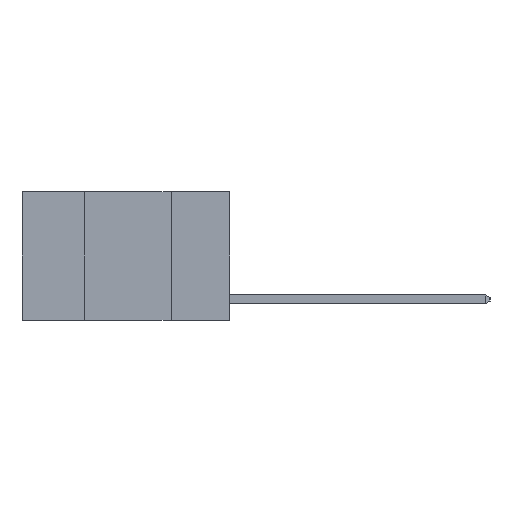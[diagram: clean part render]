
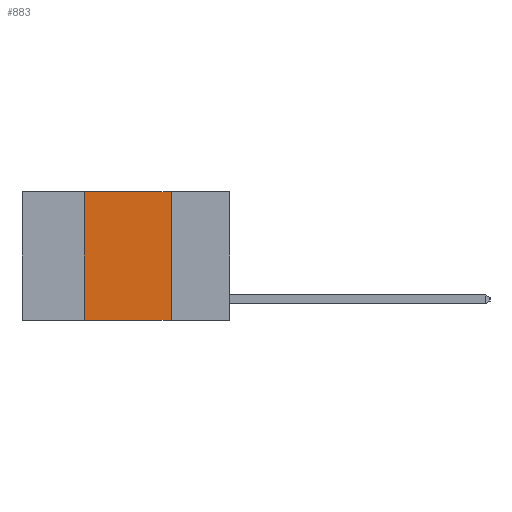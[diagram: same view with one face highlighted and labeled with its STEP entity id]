
A CAD part, left-side view. The second image highlights one B-rep face of the part: STEP entity #883.
In plain terms, the highlighted planar face has unit normal (-1, 0, 0).
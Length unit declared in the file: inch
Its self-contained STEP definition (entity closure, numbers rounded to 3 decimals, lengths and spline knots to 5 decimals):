
#25 = LINE ( 'NONE', #2860, #266 ) ;
#266 = VECTOR ( 'NONE', #7076, 39.37008 ) ;
#391 = VERTEX_POINT ( 'NONE', #4552 ) ;
#779 = CARTESIAN_POINT ( 'NONE',  ( 0., 0.17, 0. ) ) ;
#883 = ADVANCED_FACE ( 'NONE', ( #3586 ), #3807, .F. ) ;
#1099 = ORIENTED_EDGE ( 'NONE', *, *, #2950, .F. ) ;
#1114 = VERTEX_POINT ( 'NONE', #779 ) ;
#1129 = ORIENTED_EDGE ( 'NONE', *, *, #2353, .F. ) ;
#1138 = ORIENTED_EDGE ( 'NONE', *, *, #4834, .F. ) ;
#1159 = ORIENTED_EDGE ( 'NONE', *, *, #6149, .T. ) ;
#1389 = VERTEX_POINT ( 'NONE', #4564 ) ;
#2198 = AXIS2_PLACEMENT_3D ( 'NONE', #8016, #5359, #7783 ) ;
#2353 = EDGE_CURVE ( 'NONE', #5179, #1114, #6634, .T. ) ;
#2663 = VECTOR ( 'NONE', #3576, 39.37008 ) ;
#2860 = CARTESIAN_POINT ( 'NONE',  ( 0., 0.17, 0. ) ) ;
#2915 = CARTESIAN_POINT ( 'NONE',  ( 0., 0.42, 0. ) ) ;
#2950 = EDGE_CURVE ( 'NONE', #1114, #1389, #25, .T. ) ;
#3290 = CARTESIAN_POINT ( 'NONE',  ( 0., 0.42, 0. ) ) ;
#3499 = CARTESIAN_POINT ( 'NONE',  ( 0., 0.6, -0.37 ) ) ;
#3576 = DIRECTION ( 'NONE',  ( 0., 0., 1. ) ) ;
#3586 = FACE_OUTER_BOUND ( 'NONE', #4566, .T. ) ;
#3807 = PLANE ( 'NONE',  #2198 ) ;
#3913 = VECTOR ( 'NONE', #7062, 39.37008 ) ;
#4552 = CARTESIAN_POINT ( 'NONE',  ( 0., 0.42, -0.37 ) ) ;
#4564 = CARTESIAN_POINT ( 'NONE',  ( 0., 0.17, -0.37 ) ) ;
#4566 = EDGE_LOOP ( 'NONE', ( #1099, #1129, #1138, #1159 ) ) ;
#4834 = EDGE_CURVE ( 'NONE', #391, #5179, #5997, .T. ) ;
#5179 = VERTEX_POINT ( 'NONE', #3290 ) ;
#5359 = DIRECTION ( 'NONE',  ( 1., 0., 0. ) ) ;
#5884 = DIRECTION ( 'NONE',  ( 0., -1., 0. ) ) ;
#5970 = CARTESIAN_POINT ( 'NONE',  ( 0., 0.6, 0. ) ) ;
#5997 = LINE ( 'NONE', #2915, #2663 ) ;
#6149 = EDGE_CURVE ( 'NONE', #391, #1389, #7016, .T. ) ;
#6634 = LINE ( 'NONE', #5970, #7937 ) ;
#7016 = LINE ( 'NONE', #3499, #3913 ) ;
#7062 = DIRECTION ( 'NONE',  ( 0., -1., 0. ) ) ;
#7076 = DIRECTION ( 'NONE',  ( 0., 0., -1. ) ) ;
#7783 = DIRECTION ( 'NONE',  ( 0., 0., -1. ) ) ;
#7937 = VECTOR ( 'NONE', #5884, 39.37008 ) ;
#8016 = CARTESIAN_POINT ( 'NONE',  ( 0., 0.6, 0. ) ) ;
